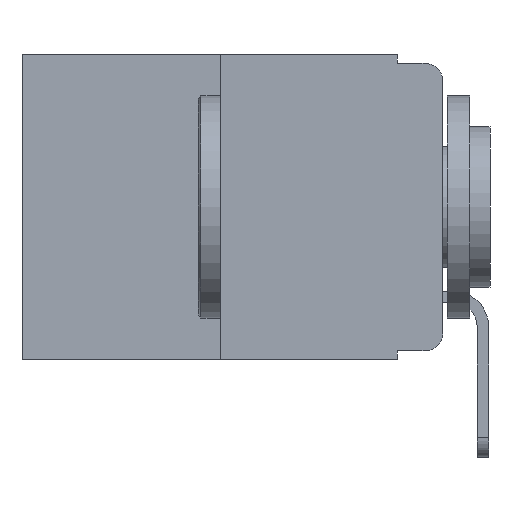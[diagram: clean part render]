
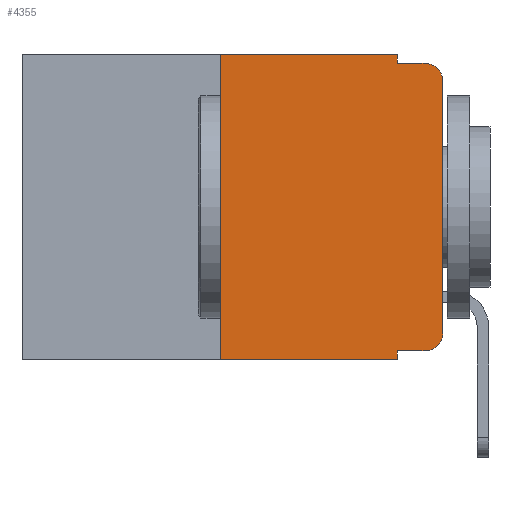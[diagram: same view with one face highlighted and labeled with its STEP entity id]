
A CAD part, left-side view. The second image highlights one B-rep face of the part: STEP entity #4355.
In plain terms, the highlighted planar face has unit normal (-1, 0, 0).
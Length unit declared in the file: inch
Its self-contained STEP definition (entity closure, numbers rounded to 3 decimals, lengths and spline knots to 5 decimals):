
#403 = LINE ( 'NONE', #12182, #8684 ) ;
#686 = EDGE_CURVE ( 'NONE', #6251, #2738, #3796, .T. ) ;
#967 = VERTEX_POINT ( 'NONE', #2826 ) ;
#1535 = ORIENTED_EDGE ( 'NONE', *, *, #686, .T. ) ;
#1651 = VERTEX_POINT ( 'NONE', #12389 ) ;
#1654 = CARTESIAN_POINT ( 'NONE',  ( 0., 0.051, 0. ) ) ;
#1735 = CARTESIAN_POINT ( 'NONE',  ( 0., 0.473, 0. ) ) ;
#1926 = VECTOR ( 'NONE', #12569, 39.37008 ) ;
#2344 = ORIENTED_EDGE ( 'NONE', *, *, #5742, .F. ) ;
#2579 = EDGE_CURVE ( 'NONE', #8963, #967, #4748, .T. ) ;
#2738 = VERTEX_POINT ( 'NONE', #12475 ) ;
#2826 = CARTESIAN_POINT ( 'NONE',  ( 0., 0.02, -0.333 ) ) ;
#3029 = EDGE_CURVE ( 'NONE', #9737, #4156, #12892, .T. ) ;
#3354 = ORIENTED_EDGE ( 'NONE', *, *, #6411, .F. ) ;
#3440 = LINE ( 'NONE', #1654, #5879 ) ;
#3443 = LINE ( 'NONE', #5057, #5880 ) ;
#3461 = VECTOR ( 'NONE', #12592, 39.37008 ) ;
#3581 = CARTESIAN_POINT ( 'NONE',  ( 0., 0.051, -0.01 ) ) ;
#3796 = LINE ( 'NONE', #4771, #3461 ) ;
#3821 = DIRECTION ( 'NONE',  ( -1., 0., 0. ) ) ;
#4156 = VERTEX_POINT ( 'NONE', #11347 ) ;
#4355 = ADVANCED_FACE ( 'NONE', ( #5285 ), #5048, .F. ) ;
#4520 = CARTESIAN_POINT ( 'NONE',  ( 0., 0.051, -0.333 ) ) ;
#4748 = LINE ( 'NONE', #7492, #1926 ) ;
#4750 = AXIS2_PLACEMENT_3D ( 'NONE', #6093, #13249, #7112 ) ;
#4771 = CARTESIAN_POINT ( 'NONE',  ( 0., 0.473, -0.343 ) ) ;
#4827 = DIRECTION ( 'NONE',  ( 0., 0., -1. ) ) ;
#4842 = DIRECTION ( 'NONE',  ( 0., 0., -1. ) ) ;
#4935 = DIRECTION ( 'NONE',  ( 0., -1., 0. ) ) ;
#5048 = PLANE ( 'NONE',  #5137 ) ;
#5057 = CARTESIAN_POINT ( 'NONE',  ( 0., 0.25, 0. ) ) ;
#5137 = AXIS2_PLACEMENT_3D ( 'NONE', #7251, #9802, #4827 ) ;
#5161 = CIRCLE ( 'NONE', #9247, 0.02 ) ;
#5285 = FACE_OUTER_BOUND ( 'NONE', #6614, .T. ) ;
#5356 = CARTESIAN_POINT ( 'NONE',  ( 0., 0., -0.313 ) ) ;
#5448 = VERTEX_POINT ( 'NONE', #12675 ) ;
#5483 = ORIENTED_EDGE ( 'NONE', *, *, #2579, .T. ) ;
#5654 = EDGE_CURVE ( 'NONE', #8963, #2738, #3440, .T. ) ;
#5742 = EDGE_CURVE ( 'NONE', #1651, #5448, #13076, .T. ) ;
#5855 = CARTESIAN_POINT ( 'NONE',  ( 0., 0.25, -0.343 ) ) ;
#5879 = VECTOR ( 'NONE', #4842, 39.37008 ) ;
#5880 = VECTOR ( 'NONE', #7100, 39.37008 ) ;
#6030 = DIRECTION ( 'NONE',  ( 0., 0., 1. ) ) ;
#6085 = EDGE_CURVE ( 'NONE', #5448, #9737, #9178, .T. ) ;
#6093 = CARTESIAN_POINT ( 'NONE',  ( 0., 0.02, -0.313 ) ) ;
#6251 = VERTEX_POINT ( 'NONE', #5855 ) ;
#6411 = EDGE_CURVE ( 'NONE', #6251, #1651, #3443, .T. ) ;
#6440 = ORIENTED_EDGE ( 'NONE', *, *, #8787, .T. ) ;
#6500 = VECTOR ( 'NONE', #9477, 39.37008 ) ;
#6614 = EDGE_LOOP ( 'NONE', ( #10884, #9116, #12851, #6905, #2344, #3354, #1535, #12382, #5483, #6440 ) ) ;
#6905 = ORIENTED_EDGE ( 'NONE', *, *, #6085, .F. ) ;
#7100 = DIRECTION ( 'NONE',  ( 0., 0., 1. ) ) ;
#7112 = DIRECTION ( 'NONE',  ( 0., 0., -1. ) ) ;
#7251 = CARTESIAN_POINT ( 'NONE',  ( 0., 0.473, 0. ) ) ;
#7375 = DIRECTION ( 'NONE',  ( 0., -1., 0. ) ) ;
#7492 = CARTESIAN_POINT ( 'NONE',  ( 0., 0.051, -0.333 ) ) ;
#7624 = VECTOR ( 'NONE', #4935, 39.37008 ) ;
#7697 = CARTESIAN_POINT ( 'NONE',  ( 0., 0., -0.03 ) ) ;
#7710 = CARTESIAN_POINT ( 'NONE',  ( 0., 0.051, -0.01 ) ) ;
#8023 = EDGE_CURVE ( 'NONE', #8269, #11209, #403, .T. ) ;
#8269 = VERTEX_POINT ( 'NONE', #5356 ) ;
#8684 = VECTOR ( 'NONE', #6030, 39.37008 ) ;
#8787 = EDGE_CURVE ( 'NONE', #967, #8269, #10247, .T. ) ;
#8963 = VERTEX_POINT ( 'NONE', #4520 ) ;
#9116 = ORIENTED_EDGE ( 'NONE', *, *, #9216, .T. ) ;
#9178 = LINE ( 'NONE', #12583, #6500 ) ;
#9216 = EDGE_CURVE ( 'NONE', #11209, #4156, #5161, .T. ) ;
#9247 = AXIS2_PLACEMENT_3D ( 'NONE', #9928, #3821, #10969 ) ;
#9477 = DIRECTION ( 'NONE',  ( 0., 0., -1. ) ) ;
#9737 = VERTEX_POINT ( 'NONE', #3581 ) ;
#9802 = DIRECTION ( 'NONE',  ( 1., 0., 0. ) ) ;
#9928 = CARTESIAN_POINT ( 'NONE',  ( 0., 0.02, -0.03 ) ) ;
#10120 = VECTOR ( 'NONE', #7375, 39.37008 ) ;
#10247 = CIRCLE ( 'NONE', #4750, 0.02 ) ;
#10884 = ORIENTED_EDGE ( 'NONE', *, *, #8023, .T. ) ;
#10969 = DIRECTION ( 'NONE',  ( 0., 0., -1. ) ) ;
#11209 = VERTEX_POINT ( 'NONE', #7697 ) ;
#11347 = CARTESIAN_POINT ( 'NONE',  ( 0., 0.02, -0.01 ) ) ;
#12182 = CARTESIAN_POINT ( 'NONE',  ( 0., 0., 0. ) ) ;
#12382 = ORIENTED_EDGE ( 'NONE', *, *, #5654, .F. ) ;
#12389 = CARTESIAN_POINT ( 'NONE',  ( 0., 0.25, 0. ) ) ;
#12475 = CARTESIAN_POINT ( 'NONE',  ( 0., 0.051, -0.343 ) ) ;
#12569 = DIRECTION ( 'NONE',  ( 0., -1., 0. ) ) ;
#12583 = CARTESIAN_POINT ( 'NONE',  ( 0., 0.051, 0. ) ) ;
#12592 = DIRECTION ( 'NONE',  ( 0., -1., 0. ) ) ;
#12675 = CARTESIAN_POINT ( 'NONE',  ( 0., 0.051, 0. ) ) ;
#12851 = ORIENTED_EDGE ( 'NONE', *, *, #3029, .F. ) ;
#12892 = LINE ( 'NONE', #7710, #10120 ) ;
#13076 = LINE ( 'NONE', #1735, #7624 ) ;
#13249 = DIRECTION ( 'NONE',  ( -1., 0., 0. ) ) ;
